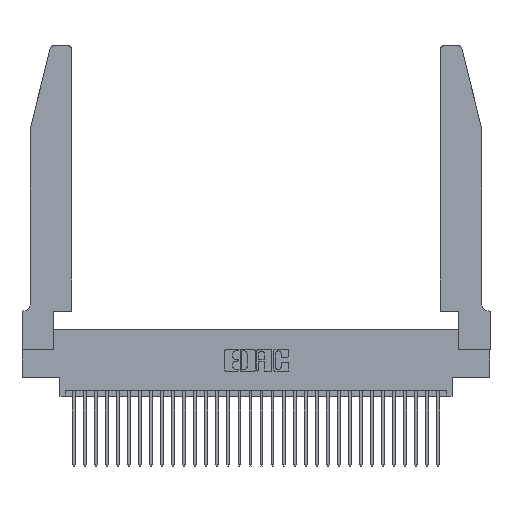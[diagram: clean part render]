
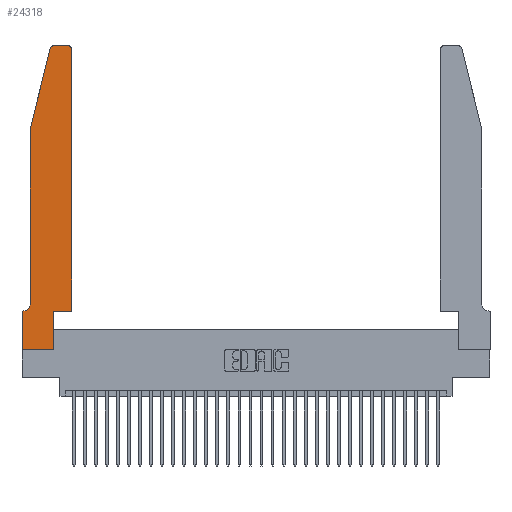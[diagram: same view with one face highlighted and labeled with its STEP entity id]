
A CAD part, top view. The second image highlights one B-rep face of the part: STEP entity #24318.
In plain terms, the highlighted planar face has unit normal (0, 0, 1).
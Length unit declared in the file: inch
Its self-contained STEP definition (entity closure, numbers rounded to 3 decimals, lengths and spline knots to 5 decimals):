
#183 = ORIENTED_EDGE ( 'NONE', *, *, #19357, .T. ) ;
#206 = VECTOR ( 'NONE', #14970, 39.37008 ) ;
#518 = CARTESIAN_POINT ( 'NONE',  ( 0.0755, 0.35, 0.37 ) ) ;
#628 = CARTESIAN_POINT ( 'NONE',  ( 0.4505, 0.35, 0.37 ) ) ;
#845 = ORIENTED_EDGE ( 'NONE', *, *, #16318, .T. ) ;
#910 = CARTESIAN_POINT ( 'NONE',  ( 0.0055, 0.35, 0.37 ) ) ;
#990 = DIRECTION ( 'NONE',  ( 1., 0., 0. ) ) ;
#1483 = EDGE_CURVE ( 'NONE', #23527, #8087, #30274, .T. ) ;
#1646 = CARTESIAN_POINT ( 'NONE',  ( 0.2605, 2.75, 0.37 ) ) ;
#1883 = EDGE_CURVE ( 'NONE', #21239, #24093, #23182, .T. ) ;
#1974 = AXIS2_PLACEMENT_3D ( 'NONE', #18815, #23787, #990 ) ;
#2821 = ORIENTED_EDGE ( 'NONE', *, *, #1483, .T. ) ;
#2972 = CARTESIAN_POINT ( 'NONE',  ( 0.0755, 2., 0.37 ) ) ;
#3355 = DIRECTION ( 'NONE',  ( -1., 0., 0. ) ) ;
#4278 = ORIENTED_EDGE ( 'NONE', *, *, #1883, .T. ) ;
#4896 = EDGE_CURVE ( 'NONE', #11834, #30636, #12790, .T. ) ;
#5262 = VECTOR ( 'NONE', #18425, 39.37008 ) ;
#5630 = CIRCLE ( 'NONE', #13825, 0.07 ) ;
#5908 = ORIENTED_EDGE ( 'NONE', *, *, #19852, .T. ) ;
#6524 = DIRECTION ( 'NONE',  ( -1., 0., 0. ) ) ;
#6641 = CARTESIAN_POINT ( 'NONE',  ( 0.0055, 0.42, 0.37 ) ) ;
#7152 = CARTESIAN_POINT ( 'NONE',  ( 0., 0.35, 0.37 ) ) ;
#7165 = VERTEX_POINT ( 'NONE', #27718 ) ;
#7315 = DIRECTION ( 'NONE',  ( 0., 1., 0. ) ) ;
#7724 = VECTOR ( 'NONE', #22855, 39.37008 ) ;
#7741 = DIRECTION ( 'NONE',  ( 1., 0., 0. ) ) ;
#7760 = DIRECTION ( 'NONE',  ( 0., 0., 1. ) ) ;
#8087 = VERTEX_POINT ( 'NONE', #20724 ) ;
#8439 = LINE ( 'NONE', #2972, #31723 ) ;
#8582 = ORIENTED_EDGE ( 'NONE', *, *, #20154, .T. ) ;
#8776 = VERTEX_POINT ( 'NONE', #20879 ) ;
#9450 = CARTESIAN_POINT ( 'NONE',  ( 0.0755, 0.42, 0.37 ) ) ;
#10259 = LINE ( 'NONE', #28623, #20152 ) ;
#10404 = EDGE_CURVE ( 'NONE', #22660, #7165, #10259, .T. ) ;
#10578 = ORIENTED_EDGE ( 'NONE', *, *, #13648, .T. ) ;
#11040 = LINE ( 'NONE', #20477, #30348 ) ;
#11686 = DIRECTION ( 'NONE',  ( 0., -1., 0. ) ) ;
#11729 = ORIENTED_EDGE ( 'NONE', *, *, #4896, .T. ) ;
#11834 = VERTEX_POINT ( 'NONE', #15123 ) ;
#12282 = VECTOR ( 'NONE', #7741, 39.37008 ) ;
#12633 = PLANE ( 'NONE',  #31379 ) ;
#12718 = VERTEX_POINT ( 'NONE', #910 ) ;
#12790 = LINE ( 'NONE', #23599, #5262 ) ;
#12824 = DIRECTION ( 'NONE',  ( 1., 0., 0. ) ) ;
#13487 = DIRECTION ( 'NONE',  ( 1., 0., 0. ) ) ;
#13648 = EDGE_CURVE ( 'NONE', #29654, #8776, #30203, .T. ) ;
#13825 = AXIS2_PLACEMENT_3D ( 'NONE', #6641, #21674, #6524 ) ;
#14432 = EDGE_LOOP ( 'NONE', ( #10578, #31856, #5908, #4278, #8582, #183, #2821, #845, #11729, #23834, #27826, #30658 ) ) ;
#14929 = VECTOR ( 'NONE', #11686, 39.37008 ) ;
#14970 = DIRECTION ( 'NONE',  ( 0., -1., 0. ) ) ;
#15123 = CARTESIAN_POINT ( 'NONE',  ( 0.2865, 0., 0.37 ) ) ;
#15221 = CARTESIAN_POINT ( 'NONE',  ( 0.2865, 0.35, 0.37 ) ) ;
#16076 = CARTESIAN_POINT ( 'NONE',  ( 0.25487, 2.72718, 0.37 ) ) ;
#16318 = EDGE_CURVE ( 'NONE', #8087, #11834, #11040, .T. ) ;
#16706 = VECTOR ( 'NONE', #3355, 39.37008 ) ;
#17120 = EDGE_CURVE ( 'NONE', #7165, #29654, #26360, .T. ) ;
#18404 = AXIS2_PLACEMENT_3D ( 'NONE', #32142, #27419, #22145 ) ;
#18425 = DIRECTION ( 'NONE',  ( 0., 1., 0. ) ) ;
#18815 = CARTESIAN_POINT ( 'NONE',  ( 0.284, 2.72, 0.37 ) ) ;
#19357 = EDGE_CURVE ( 'NONE', #12718, #23527, #30865, .T. ) ;
#19540 = CIRCLE ( 'NONE', #1974, 0.03 ) ;
#19852 = EDGE_CURVE ( 'NONE', #32424, #21239, #8439, .T. ) ;
#20152 = VECTOR ( 'NONE', #7315, 39.37008 ) ;
#20154 = EDGE_CURVE ( 'NONE', #24093, #12718, #5630, .T. ) ;
#20477 = CARTESIAN_POINT ( 'NONE',  ( 0., 0., 0.37 ) ) ;
#20563 = CARTESIAN_POINT ( 'NONE',  ( 0., 0.35, 0.37 ) ) ;
#20692 = CARTESIAN_POINT ( 'NONE',  ( 0.4205, 2.75, 0.37 ) ) ;
#20724 = CARTESIAN_POINT ( 'NONE',  ( 0., 0., 0.37 ) ) ;
#20879 = CARTESIAN_POINT ( 'NONE',  ( 0.284, 2.75, 0.37 ) ) ;
#21239 = VERTEX_POINT ( 'NONE', #27949 ) ;
#21674 = DIRECTION ( 'NONE',  ( 0., 0., -1. ) ) ;
#22145 = DIRECTION ( 'NONE',  ( 1., 0., 0. ) ) ;
#22643 = FACE_OUTER_BOUND ( 'NONE', #14432, .T. ) ;
#22647 = CARTESIAN_POINT ( 'NONE',  ( 0.4505, 0.35, 0.37 ) ) ;
#22660 = VERTEX_POINT ( 'NONE', #628 ) ;
#22855 = DIRECTION ( 'NONE',  ( -1., 0., 0. ) ) ;
#23182 = LINE ( 'NONE', #24023, #14929 ) ;
#23527 = VERTEX_POINT ( 'NONE', #7152 ) ;
#23599 = CARTESIAN_POINT ( 'NONE',  ( 0.2865, 0.35, 0.37 ) ) ;
#23787 = DIRECTION ( 'NONE',  ( 0., 0., 1. ) ) ;
#23805 = EDGE_CURVE ( 'NONE', #8776, #32424, #19540, .T. ) ;
#23834 = ORIENTED_EDGE ( 'NONE', *, *, #32015, .T. ) ;
#24023 = CARTESIAN_POINT ( 'NONE',  ( 0.0755, 2., 0.37 ) ) ;
#24093 = VERTEX_POINT ( 'NONE', #9450 ) ;
#24318 = ADVANCED_FACE ( 'NONE', ( #22643 ), #12633, .T. ) ;
#25693 = LINE ( 'NONE', #22647, #12282 ) ;
#26360 = CIRCLE ( 'NONE', #18404, 0.03 ) ;
#27419 = DIRECTION ( 'NONE',  ( 0., 0., 1. ) ) ;
#27718 = CARTESIAN_POINT ( 'NONE',  ( 0.4505, 2.72, 0.37 ) ) ;
#27826 = ORIENTED_EDGE ( 'NONE', *, *, #10404, .T. ) ;
#27949 = CARTESIAN_POINT ( 'NONE',  ( 0.0755, 2., 0.37 ) ) ;
#28623 = CARTESIAN_POINT ( 'NONE',  ( 0.4505, 0.35, 0.37 ) ) ;
#29654 = VERTEX_POINT ( 'NONE', #20692 ) ;
#29923 = CARTESIAN_POINT ( 'NONE',  ( 0., 0., 0.37 ) ) ;
#30203 = LINE ( 'NONE', #1646, #7724 ) ;
#30274 = LINE ( 'NONE', #29923, #206 ) ;
#30348 = VECTOR ( 'NONE', #13487, 39.37008 ) ;
#30636 = VERTEX_POINT ( 'NONE', #15221 ) ;
#30658 = ORIENTED_EDGE ( 'NONE', *, *, #17120, .T. ) ;
#30763 = DIRECTION ( 'NONE',  ( -0.239, -0.971, 0. ) ) ;
#30865 = LINE ( 'NONE', #518, #16706 ) ;
#31379 = AXIS2_PLACEMENT_3D ( 'NONE', #20563, #7760, #12824 ) ;
#31723 = VECTOR ( 'NONE', #30763, 39.37008 ) ;
#31856 = ORIENTED_EDGE ( 'NONE', *, *, #23805, .T. ) ;
#32015 = EDGE_CURVE ( 'NONE', #30636, #22660, #25693, .T. ) ;
#32142 = CARTESIAN_POINT ( 'NONE',  ( 0.4205, 2.72, 0.37 ) ) ;
#32424 = VERTEX_POINT ( 'NONE', #16076 ) ;
